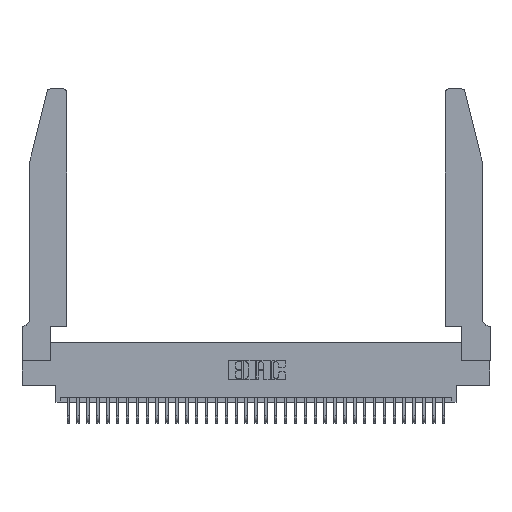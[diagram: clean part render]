
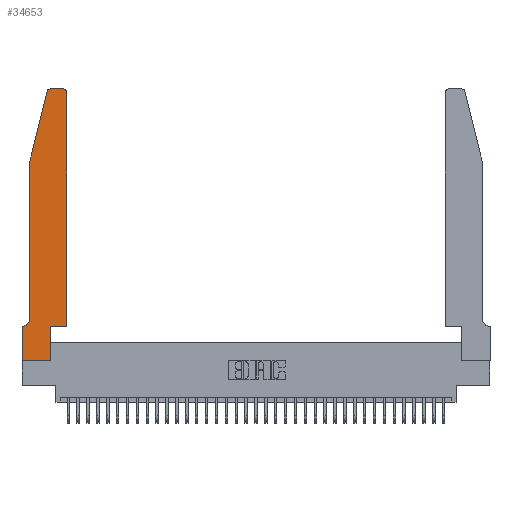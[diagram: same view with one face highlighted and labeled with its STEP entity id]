
A CAD part, top view. The second image highlights one B-rep face of the part: STEP entity #34653.
In plain terms, the highlighted planar face has unit normal (0, 0, 1).
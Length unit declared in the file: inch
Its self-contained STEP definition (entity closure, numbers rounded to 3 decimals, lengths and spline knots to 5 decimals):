
#167 = EDGE_CURVE ( 'NONE', #30106, #13308, #2636, .T. ) ;
#319 = VECTOR ( 'NONE', #20163, 39.37008 ) ;
#331 = AXIS2_PLACEMENT_3D ( 'NONE', #13544, #33603, #7857 ) ;
#397 = ORIENTED_EDGE ( 'NONE', *, *, #37033, .T. ) ;
#438 = DIRECTION ( 'NONE',  ( 0., 0., 1. ) ) ;
#447 = EDGE_CURVE ( 'NONE', #26433, #30410, #25260, .T. ) ;
#502 = AXIS2_PLACEMENT_3D ( 'NONE', #1390, #7817, #36240 ) ;
#658 = CARTESIAN_POINT ( 'NONE',  ( 0., 0., 0.37 ) ) ;
#740 = EDGE_CURVE ( 'NONE', #23763, #29824, #7526, .T. ) ;
#985 = LINE ( 'NONE', #658, #36940 ) ;
#1390 = CARTESIAN_POINT ( 'NONE',  ( 0.0055, 0.42, 0.37 ) ) ;
#1843 = CARTESIAN_POINT ( 'NONE',  ( 0.284, 2.75, 0.37 ) ) ;
#2636 = LINE ( 'NONE', #8515, #319 ) ;
#2828 = LINE ( 'NONE', #37242, #27217 ) ;
#2925 = EDGE_CURVE ( 'NONE', #32020, #18745, #15010, .T. ) ;
#3873 = VECTOR ( 'NONE', #4019, 39.37008 ) ;
#4019 = DIRECTION ( 'NONE',  ( 0., -1., 0. ) ) ;
#4087 = ORIENTED_EDGE ( 'NONE', *, *, #447, .T. ) ;
#4577 = VERTEX_POINT ( 'NONE', #1843 ) ;
#5678 = CARTESIAN_POINT ( 'NONE',  ( 0.0055, 0.35, 0.37 ) ) ;
#5846 = CARTESIAN_POINT ( 'NONE',  ( 0.0755, 0.42, 0.37 ) ) ;
#6093 = EDGE_CURVE ( 'NONE', #13308, #32020, #6678, .T. ) ;
#6350 = ORIENTED_EDGE ( 'NONE', *, *, #6093, .T. ) ;
#6678 = LINE ( 'NONE', #7207, #23062 ) ;
#7207 = CARTESIAN_POINT ( 'NONE',  ( 0.0755, 2., 0.37 ) ) ;
#7288 = CARTESIAN_POINT ( 'NONE',  ( 0.0755, 0.35, 0.37 ) ) ;
#7526 = LINE ( 'NONE', #10485, #3873 ) ;
#7623 = CARTESIAN_POINT ( 'NONE',  ( 0.4205, 2.72, 0.37 ) ) ;
#7817 = DIRECTION ( 'NONE',  ( 0., 0., -1. ) ) ;
#7857 = DIRECTION ( 'NONE',  ( 1., 0., 0. ) ) ;
#8375 = ORIENTED_EDGE ( 'NONE', *, *, #167, .T. ) ;
#8445 = EDGE_CURVE ( 'NONE', #25677, #14465, #2828, .T. ) ;
#8515 = CARTESIAN_POINT ( 'NONE',  ( 0.0755, 2., 0.37 ) ) ;
#8735 = CIRCLE ( 'NONE', #27603, 0.03 ) ;
#9404 = DIRECTION ( 'NONE',  ( 1., 0., 0. ) ) ;
#10485 = CARTESIAN_POINT ( 'NONE',  ( 0., 0., 0.37 ) ) ;
#11470 = EDGE_LOOP ( 'NONE', ( #18072, #22118, #8375, #6350, #20782, #29630, #17114, #397, #4087, #29405, #17874, #31081 ) ) ;
#12521 = LINE ( 'NONE', #24072, #13502 ) ;
#13103 = DIRECTION ( 'NONE',  ( -1., 0., 0. ) ) ;
#13308 = VERTEX_POINT ( 'NONE', #27665 ) ;
#13502 = VECTOR ( 'NONE', #32833, 39.37008 ) ;
#13544 = CARTESIAN_POINT ( 'NONE',  ( 0., 0.35, 0.37 ) ) ;
#13726 = DIRECTION ( 'NONE',  ( 0., 1., 0. ) ) ;
#14334 = FACE_OUTER_BOUND ( 'NONE', #11470, .T. ) ;
#14380 = CARTESIAN_POINT ( 'NONE',  ( 0.4505, 0.35, 0.37 ) ) ;
#14465 = VERTEX_POINT ( 'NONE', #15887 ) ;
#14792 = VECTOR ( 'NONE', #25966, 39.37008 ) ;
#14904 = EDGE_CURVE ( 'NONE', #33762, #4577, #31193, .T. ) ;
#15010 = CIRCLE ( 'NONE', #502, 0.07 ) ;
#15751 = DIRECTION ( 'NONE',  ( 1., 0., 0. ) ) ;
#15887 = CARTESIAN_POINT ( 'NONE',  ( 0.4505, 2.72, 0.37 ) ) ;
#17114 = ORIENTED_EDGE ( 'NONE', *, *, #740, .T. ) ;
#17874 = ORIENTED_EDGE ( 'NONE', *, *, #8445, .T. ) ;
#18072 = ORIENTED_EDGE ( 'NONE', *, *, #14904, .T. ) ;
#18745 = VERTEX_POINT ( 'NONE', #5678 ) ;
#19285 = DIRECTION ( 'NONE',  ( 0., 0., 1. ) ) ;
#19679 = CIRCLE ( 'NONE', #35689, 0.03 ) ;
#20163 = DIRECTION ( 'NONE',  ( -0.239, -0.971, 0. ) ) ;
#20194 = CARTESIAN_POINT ( 'NONE',  ( 0., 0., 0.37 ) ) ;
#20398 = CARTESIAN_POINT ( 'NONE',  ( 0.2865, 0.35, 0.37 ) ) ;
#20782 = ORIENTED_EDGE ( 'NONE', *, *, #2925, .T. ) ;
#21274 = EDGE_CURVE ( 'NONE', #14465, #33762, #8735, .T. ) ;
#22118 = ORIENTED_EDGE ( 'NONE', *, *, #25828, .T. ) ;
#22460 = DIRECTION ( 'NONE',  ( 1., 0., 0. ) ) ;
#22471 = CARTESIAN_POINT ( 'NONE',  ( 0.4205, 2.75, 0.37 ) ) ;
#22539 = VECTOR ( 'NONE', #37006, 39.37008 ) ;
#23062 = VECTOR ( 'NONE', #27485, 39.37008 ) ;
#23067 = VECTOR ( 'NONE', #13103, 39.37008 ) ;
#23763 = VERTEX_POINT ( 'NONE', #31225 ) ;
#24072 = CARTESIAN_POINT ( 'NONE',  ( 0.4505, 0.35, 0.37 ) ) ;
#25260 = LINE ( 'NONE', #25303, #22539 ) ;
#25303 = CARTESIAN_POINT ( 'NONE',  ( 0.2865, 0.35, 0.37 ) ) ;
#25677 = VERTEX_POINT ( 'NONE', #14380 ) ;
#25828 = EDGE_CURVE ( 'NONE', #4577, #30106, #19679, .T. ) ;
#25966 = DIRECTION ( 'NONE',  ( -1., 0., 0. ) ) ;
#26433 = VERTEX_POINT ( 'NONE', #29652 ) ;
#26664 = CARTESIAN_POINT ( 'NONE',  ( 0.284, 2.72, 0.37 ) ) ;
#27217 = VECTOR ( 'NONE', #13726, 39.37008 ) ;
#27485 = DIRECTION ( 'NONE',  ( 0., -1., 0. ) ) ;
#27603 = AXIS2_PLACEMENT_3D ( 'NONE', #7623, #19285, #22460 ) ;
#27665 = CARTESIAN_POINT ( 'NONE',  ( 0.0755, 2., 0.37 ) ) ;
#27766 = CARTESIAN_POINT ( 'NONE',  ( 0.25487, 2.72718, 0.37 ) ) ;
#27866 = PLANE ( 'NONE',  #331 ) ;
#28970 = EDGE_CURVE ( 'NONE', #18745, #23763, #30789, .T. ) ;
#29405 = ORIENTED_EDGE ( 'NONE', *, *, #29525, .T. ) ;
#29525 = EDGE_CURVE ( 'NONE', #30410, #25677, #12521, .T. ) ;
#29630 = ORIENTED_EDGE ( 'NONE', *, *, #28970, .T. ) ;
#29652 = CARTESIAN_POINT ( 'NONE',  ( 0.2865, 0., 0.37 ) ) ;
#29824 = VERTEX_POINT ( 'NONE', #20194 ) ;
#30106 = VERTEX_POINT ( 'NONE', #27766 ) ;
#30410 = VERTEX_POINT ( 'NONE', #20398 ) ;
#30789 = LINE ( 'NONE', #7288, #23067 ) ;
#31081 = ORIENTED_EDGE ( 'NONE', *, *, #21274, .T. ) ;
#31193 = LINE ( 'NONE', #36778, #14792 ) ;
#31225 = CARTESIAN_POINT ( 'NONE',  ( 0., 0.35, 0.37 ) ) ;
#32020 = VERTEX_POINT ( 'NONE', #5846 ) ;
#32833 = DIRECTION ( 'NONE',  ( 1., 0., 0. ) ) ;
#33603 = DIRECTION ( 'NONE',  ( 0., 0., 1. ) ) ;
#33762 = VERTEX_POINT ( 'NONE', #22471 ) ;
#34653 = ADVANCED_FACE ( 'NONE', ( #14334 ), #27866, .T. ) ;
#35689 = AXIS2_PLACEMENT_3D ( 'NONE', #26664, #438, #9404 ) ;
#36240 = DIRECTION ( 'NONE',  ( -1., 0., 0. ) ) ;
#36778 = CARTESIAN_POINT ( 'NONE',  ( 0.2605, 2.75, 0.37 ) ) ;
#36940 = VECTOR ( 'NONE', #15751, 39.37008 ) ;
#37006 = DIRECTION ( 'NONE',  ( 0., 1., 0. ) ) ;
#37033 = EDGE_CURVE ( 'NONE', #29824, #26433, #985, .T. ) ;
#37242 = CARTESIAN_POINT ( 'NONE',  ( 0.4505, 0.35, 0.37 ) ) ;
